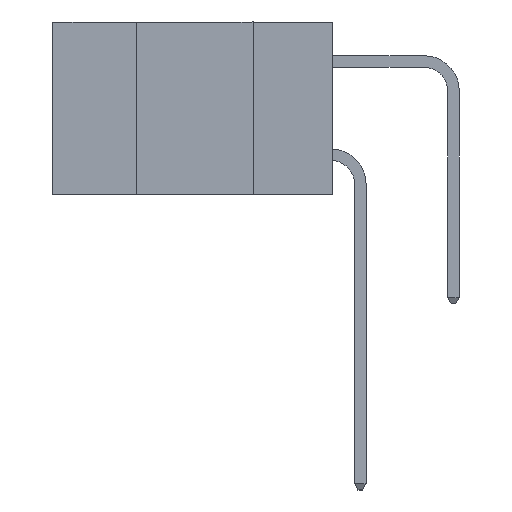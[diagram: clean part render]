
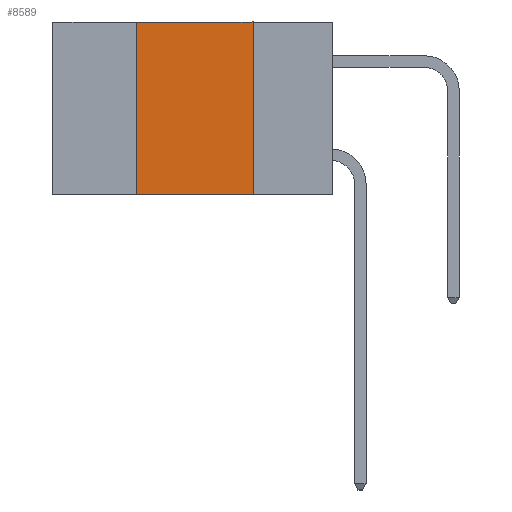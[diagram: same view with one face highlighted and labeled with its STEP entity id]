
A CAD part, left-side view. The second image highlights one B-rep face of the part: STEP entity #8589.
In plain terms, the highlighted planar face has unit normal (-1, 0, 0).
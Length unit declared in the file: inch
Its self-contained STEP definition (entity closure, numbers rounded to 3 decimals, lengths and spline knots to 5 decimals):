
#169 = VERTEX_POINT ( 'NONE', #10718 ) ;
#1635 = VECTOR ( 'NONE', #2871, 39.37008 ) ;
#2127 = VECTOR ( 'NONE', #4487, 39.37008 ) ;
#2455 = AXIS2_PLACEMENT_3D ( 'NONE', #4151, #4138, #4126 ) ;
#2871 = DIRECTION ( 'NONE',  ( 0., -1., 0. ) ) ;
#2891 = CARTESIAN_POINT ( 'NONE',  ( 0., 0.6, 0. ) ) ;
#3552 = CARTESIAN_POINT ( 'NONE',  ( 0., 0.42, -0.37 ) ) ;
#3770 = LINE ( 'NONE', #12173, #6188 ) ;
#4117 = ORIENTED_EDGE ( 'NONE', *, *, #11028, .F. ) ;
#4126 = DIRECTION ( 'NONE',  ( 0., 0., -1. ) ) ;
#4138 = DIRECTION ( 'NONE',  ( 1., 0., 0. ) ) ;
#4151 = CARTESIAN_POINT ( 'NONE',  ( 0., 0.6, 0. ) ) ;
#4179 = PLANE ( 'NONE',  #2455 ) ;
#4352 = FACE_OUTER_BOUND ( 'NONE', #5648, .T. ) ;
#4487 = DIRECTION ( 'NONE',  ( 0., -1., 0. ) ) ;
#4520 = CARTESIAN_POINT ( 'NONE',  ( 0., 0.6, -0.37 ) ) ;
#5226 = LINE ( 'NONE', #3552, #13032 ) ;
#5458 = VERTEX_POINT ( 'NONE', #8925 ) ;
#5648 = EDGE_LOOP ( 'NONE', ( #4117, #10689, #11935, #8387 ) ) ;
#6188 = VECTOR ( 'NONE', #11176, 39.37008 ) ;
#6214 = EDGE_CURVE ( 'NONE', #7918, #169, #12080, .T. ) ;
#6662 = DIRECTION ( 'NONE',  ( 0., 0., 1. ) ) ;
#7397 = VERTEX_POINT ( 'NONE', #13350 ) ;
#7918 = VERTEX_POINT ( 'NONE', #8907 ) ;
#8387 = ORIENTED_EDGE ( 'NONE', *, *, #8553, .T. ) ;
#8553 = EDGE_CURVE ( 'NONE', #5458, #7397, #10435, .T. ) ;
#8589 = ADVANCED_FACE ( 'NONE', ( #4352 ), #4179, .F. ) ;
#8907 = CARTESIAN_POINT ( 'NONE',  ( 0., 0.42, 0. ) ) ;
#8925 = CARTESIAN_POINT ( 'NONE',  ( 0., 0.42, -0.37 ) ) ;
#10435 = LINE ( 'NONE', #4520, #2127 ) ;
#10689 = ORIENTED_EDGE ( 'NONE', *, *, #6214, .F. ) ;
#10718 = CARTESIAN_POINT ( 'NONE',  ( 0., 0.17, 0. ) ) ;
#11028 = EDGE_CURVE ( 'NONE', #169, #7397, #3770, .T. ) ;
#11176 = DIRECTION ( 'NONE',  ( 0., 0., -1. ) ) ;
#11935 = ORIENTED_EDGE ( 'NONE', *, *, #12646, .F. ) ;
#12080 = LINE ( 'NONE', #2891, #1635 ) ;
#12173 = CARTESIAN_POINT ( 'NONE',  ( 0., 0.17, -0.37 ) ) ;
#12646 = EDGE_CURVE ( 'NONE', #5458, #7918, #5226, .T. ) ;
#13032 = VECTOR ( 'NONE', #6662, 39.37008 ) ;
#13350 = CARTESIAN_POINT ( 'NONE',  ( 0., 0.17, -0.37 ) ) ;
